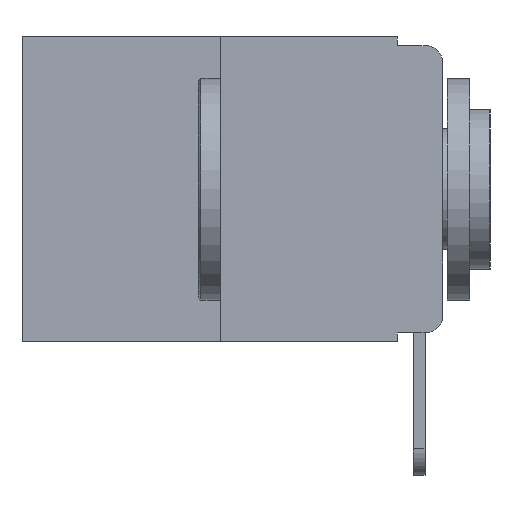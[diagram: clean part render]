
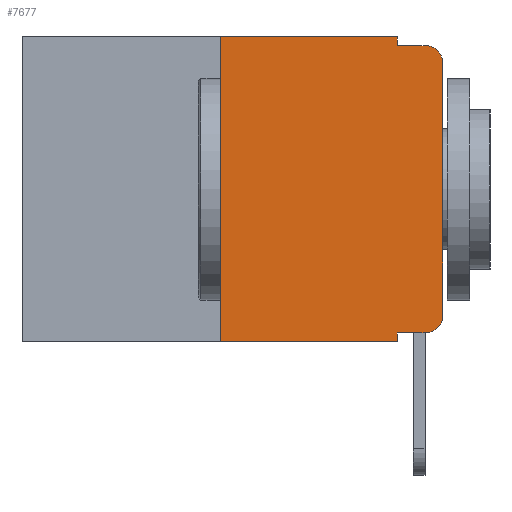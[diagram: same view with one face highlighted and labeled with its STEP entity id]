
A CAD part, left-side view. The second image highlights one B-rep face of the part: STEP entity #7677.
In plain terms, the highlighted planar face has unit normal (-1, 0, 0).
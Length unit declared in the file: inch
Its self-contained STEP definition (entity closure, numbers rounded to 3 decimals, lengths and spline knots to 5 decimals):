
#888 = CARTESIAN_POINT ( 'NONE',  ( 0., 0., -0.03 ) ) ;
#927 = LINE ( 'NONE', #1939, #12648 ) ;
#1097 = VERTEX_POINT ( 'NONE', #3303 ) ;
#1285 = LINE ( 'NONE', #6480, #9949 ) ;
#1364 = AXIS2_PLACEMENT_3D ( 'NONE', #6579, #1467, #5309 ) ;
#1467 = DIRECTION ( 'NONE',  ( 1., 0., 0. ) ) ;
#1790 = CARTESIAN_POINT ( 'NONE',  ( 0., 0.051, 0. ) ) ;
#1848 = VERTEX_POINT ( 'NONE', #14171 ) ;
#1939 = CARTESIAN_POINT ( 'NONE',  ( 0., 0.051, -0.01 ) ) ;
#2247 = VERTEX_POINT ( 'NONE', #7972 ) ;
#2394 = CARTESIAN_POINT ( 'NONE',  ( 0., 0.02, -0.313 ) ) ;
#2550 = LINE ( 'NONE', #1790, #7982 ) ;
#2606 = ORIENTED_EDGE ( 'NONE', *, *, #2977, .T. ) ;
#2731 = FACE_OUTER_BOUND ( 'NONE', #16433, .T. ) ;
#2905 = PLANE ( 'NONE',  #1364 ) ;
#2977 = EDGE_CURVE ( 'NONE', #4113, #12920, #8397, .T. ) ;
#3043 = LINE ( 'NONE', #7230, #15918 ) ;
#3163 = DIRECTION ( 'NONE',  ( -1., 0., 0. ) ) ;
#3193 = CARTESIAN_POINT ( 'NONE',  ( 0., 0.473, 0. ) ) ;
#3303 = CARTESIAN_POINT ( 'NONE',  ( 0., 0., -0.313 ) ) ;
#4003 = DIRECTION ( 'NONE',  ( 0., 0., -1. ) ) ;
#4070 = ORIENTED_EDGE ( 'NONE', *, *, #5816, .T. ) ;
#4113 = VERTEX_POINT ( 'NONE', #888 ) ;
#4800 = ORIENTED_EDGE ( 'NONE', *, *, #15427, .T. ) ;
#4931 = VERTEX_POINT ( 'NONE', #7913 ) ;
#4937 = EDGE_CURVE ( 'NONE', #2247, #14060, #3043, .T. ) ;
#5104 = ORIENTED_EDGE ( 'NONE', *, *, #5578, .T. ) ;
#5237 = ORIENTED_EDGE ( 'NONE', *, *, #10969, .F. ) ;
#5309 = DIRECTION ( 'NONE',  ( 0., 0., -1. ) ) ;
#5578 = EDGE_CURVE ( 'NONE', #2247, #14605, #9145, .T. ) ;
#5589 = CARTESIAN_POINT ( 'NONE',  ( 0., 0.051, -0.343 ) ) ;
#5749 = VERTEX_POINT ( 'NONE', #11255 ) ;
#5768 = LINE ( 'NONE', #3193, #8991 ) ;
#5816 = EDGE_CURVE ( 'NONE', #5749, #1848, #7464, .T. ) ;
#5889 = AXIS2_PLACEMENT_3D ( 'NONE', #2394, #7607, #12755 ) ;
#6125 = ORIENTED_EDGE ( 'NONE', *, *, #15522, .F. ) ;
#6480 = CARTESIAN_POINT ( 'NONE',  ( 0., 0., 0. ) ) ;
#6579 = CARTESIAN_POINT ( 'NONE',  ( 0., 0.473, 0. ) ) ;
#7230 = CARTESIAN_POINT ( 'NONE',  ( 0., 0.25, 0. ) ) ;
#7464 = LINE ( 'NONE', #8386, #15910 ) ;
#7607 = DIRECTION ( 'NONE',  ( -1., 0., 0. ) ) ;
#7677 = ADVANCED_FACE ( 'NONE', ( #2731 ), #2905, .F. ) ;
#7913 = CARTESIAN_POINT ( 'NONE',  ( 0., 0.051, 0. ) ) ;
#7972 = CARTESIAN_POINT ( 'NONE',  ( 0., 0.25, -0.343 ) ) ;
#7982 = VECTOR ( 'NONE', #4003, 39.37008 ) ;
#8015 = VECTOR ( 'NONE', #15689, 39.37008 ) ;
#8386 = CARTESIAN_POINT ( 'NONE',  ( 0., 0.051, -0.333 ) ) ;
#8397 = CIRCLE ( 'NONE', #9480, 0.02 ) ;
#8706 = EDGE_CURVE ( 'NONE', #14060, #4931, #5768, .T. ) ;
#8991 = VECTOR ( 'NONE', #13534, 39.37008 ) ;
#9145 = LINE ( 'NONE', #10173, #13022 ) ;
#9358 = LINE ( 'NONE', #9605, #8015 ) ;
#9480 = AXIS2_PLACEMENT_3D ( 'NONE', #14770, #3163, #13503 ) ;
#9595 = DIRECTION ( 'NONE',  ( 0., 0., 1. ) ) ;
#9605 = CARTESIAN_POINT ( 'NONE',  ( 0., 0.051, 0. ) ) ;
#9949 = VECTOR ( 'NONE', #11646, 39.37008 ) ;
#10173 = CARTESIAN_POINT ( 'NONE',  ( 0., 0.473, -0.343 ) ) ;
#10708 = DIRECTION ( 'NONE',  ( 0., -1., 0. ) ) ;
#10756 = CIRCLE ( 'NONE', #5889, 0.02 ) ;
#10969 = EDGE_CURVE ( 'NONE', #4931, #14336, #2550, .T. ) ;
#11004 = DIRECTION ( 'NONE',  ( 0., -1., 0. ) ) ;
#11255 = CARTESIAN_POINT ( 'NONE',  ( 0., 0.051, -0.333 ) ) ;
#11523 = CARTESIAN_POINT ( 'NONE',  ( 0., 0.051, -0.01 ) ) ;
#11646 = DIRECTION ( 'NONE',  ( 0., 0., 1. ) ) ;
#11804 = ORIENTED_EDGE ( 'NONE', *, *, #8706, .F. ) ;
#11956 = CARTESIAN_POINT ( 'NONE',  ( 0., 0.02, -0.01 ) ) ;
#12648 = VECTOR ( 'NONE', #10708, 39.37008 ) ;
#12755 = DIRECTION ( 'NONE',  ( 0., 0., -1. ) ) ;
#12920 = VERTEX_POINT ( 'NONE', #11956 ) ;
#13022 = VECTOR ( 'NONE', #13967, 39.37008 ) ;
#13353 = ORIENTED_EDGE ( 'NONE', *, *, #16588, .T. ) ;
#13503 = DIRECTION ( 'NONE',  ( 0., 0., -1. ) ) ;
#13534 = DIRECTION ( 'NONE',  ( 0., -1., 0. ) ) ;
#13591 = EDGE_CURVE ( 'NONE', #5749, #14605, #9358, .T. ) ;
#13967 = DIRECTION ( 'NONE',  ( 0., -1., 0. ) ) ;
#14060 = VERTEX_POINT ( 'NONE', #14641 ) ;
#14157 = ORIENTED_EDGE ( 'NONE', *, *, #13591, .F. ) ;
#14171 = CARTESIAN_POINT ( 'NONE',  ( 0., 0.02, -0.333 ) ) ;
#14193 = ORIENTED_EDGE ( 'NONE', *, *, #4937, .F. ) ;
#14336 = VERTEX_POINT ( 'NONE', #11523 ) ;
#14605 = VERTEX_POINT ( 'NONE', #5589 ) ;
#14641 = CARTESIAN_POINT ( 'NONE',  ( 0., 0.25, 0. ) ) ;
#14770 = CARTESIAN_POINT ( 'NONE',  ( 0., 0.02, -0.03 ) ) ;
#15427 = EDGE_CURVE ( 'NONE', #1097, #4113, #1285, .T. ) ;
#15522 = EDGE_CURVE ( 'NONE', #14336, #12920, #927, .T. ) ;
#15689 = DIRECTION ( 'NONE',  ( 0., 0., -1. ) ) ;
#15910 = VECTOR ( 'NONE', #11004, 39.37008 ) ;
#15918 = VECTOR ( 'NONE', #9595, 39.37008 ) ;
#16433 = EDGE_LOOP ( 'NONE', ( #4800, #2606, #6125, #5237, #11804, #14193, #5104, #14157, #4070, #13353 ) ) ;
#16588 = EDGE_CURVE ( 'NONE', #1848, #1097, #10756, .T. ) ;
